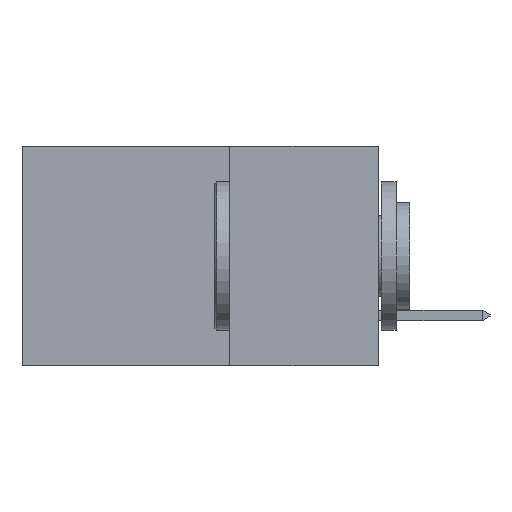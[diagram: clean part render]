
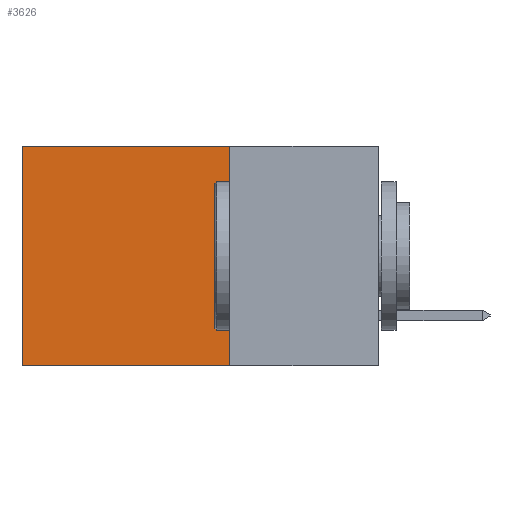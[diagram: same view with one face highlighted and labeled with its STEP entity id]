
A CAD part, left-side view. The second image highlights one B-rep face of the part: STEP entity #3626.
In plain terms, the highlighted planar face has unit normal (-1, 0, 0).
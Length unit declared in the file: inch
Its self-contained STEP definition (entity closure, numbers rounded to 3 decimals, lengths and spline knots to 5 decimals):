
#65 = CARTESIAN_POINT ( 'NONE',  ( 0.298, 0.25, -0.37 ) ) ;
#836 = ORIENTED_EDGE ( 'NONE', *, *, #17893, .F. ) ;
#1522 = LINE ( 'NONE', #2493, #18254 ) ;
#1903 = EDGE_CURVE ( 'NONE', #4703, #18599, #11554, .T. ) ;
#2493 = CARTESIAN_POINT ( 'NONE',  ( 0.298, 0.6, 0. ) ) ;
#2502 = DIRECTION ( 'NONE',  ( 0., 0., -1. ) ) ;
#2828 = FACE_OUTER_BOUND ( 'NONE', #4245, .T. ) ;
#3054 = CARTESIAN_POINT ( 'NONE',  ( 0.298, 0.25, 0. ) ) ;
#3185 = ORIENTED_EDGE ( 'NONE', *, *, #1903, .T. ) ;
#3565 = VERTEX_POINT ( 'NONE', #14821 ) ;
#3626 = ADVANCED_FACE ( 'NONE', ( #2828 ), #18429, .F. ) ;
#3678 = VECTOR ( 'NONE', #17555, 39.37008 ) ;
#4198 = EDGE_CURVE ( 'NONE', #18599, #3565, #1522, .T. ) ;
#4245 = EDGE_LOOP ( 'NONE', ( #15793, #17507, #836, #3185 ) ) ;
#4703 = VERTEX_POINT ( 'NONE', #20264 ) ;
#7183 = CARTESIAN_POINT ( 'NONE',  ( 0.298, 0.25, -0.37 ) ) ;
#8598 = LINE ( 'NONE', #3054, #12730 ) ;
#11180 = DIRECTION ( 'NONE',  ( 0., 1., 0. ) ) ;
#11554 = LINE ( 'NONE', #19436, #3678 ) ;
#12730 = VECTOR ( 'NONE', #14095, 39.37008 ) ;
#14095 = DIRECTION ( 'NONE',  ( 0., 0., -1. ) ) ;
#14559 = CARTESIAN_POINT ( 'NONE',  ( 0.298, 0.6, 0. ) ) ;
#14821 = CARTESIAN_POINT ( 'NONE',  ( 0.298, 0.6, -0.37 ) ) ;
#15094 = EDGE_CURVE ( 'NONE', #20099, #3565, #18907, .T. ) ;
#15341 = VECTOR ( 'NONE', #11180, 39.37008 ) ;
#15793 = ORIENTED_EDGE ( 'NONE', *, *, #4198, .T. ) ;
#17507 = ORIENTED_EDGE ( 'NONE', *, *, #15094, .F. ) ;
#17513 = DIRECTION ( 'NONE',  ( 0., 0., -1. ) ) ;
#17517 = DIRECTION ( 'NONE',  ( 1., 0., 0. ) ) ;
#17555 = DIRECTION ( 'NONE',  ( 0., 1., 0. ) ) ;
#17579 = CARTESIAN_POINT ( 'NONE',  ( 0.298, 0.25, 0. ) ) ;
#17893 = EDGE_CURVE ( 'NONE', #4703, #20099, #8598, .T. ) ;
#18254 = VECTOR ( 'NONE', #2502, 39.37008 ) ;
#18429 = PLANE ( 'NONE',  #19594 ) ;
#18599 = VERTEX_POINT ( 'NONE', #14559 ) ;
#18907 = LINE ( 'NONE', #65, #15341 ) ;
#19436 = CARTESIAN_POINT ( 'NONE',  ( 0.298, 0.25, 0. ) ) ;
#19594 = AXIS2_PLACEMENT_3D ( 'NONE', #17579, #17517, #17513 ) ;
#20099 = VERTEX_POINT ( 'NONE', #7183 ) ;
#20264 = CARTESIAN_POINT ( 'NONE',  ( 0.298, 0.25, 0. ) ) ;
